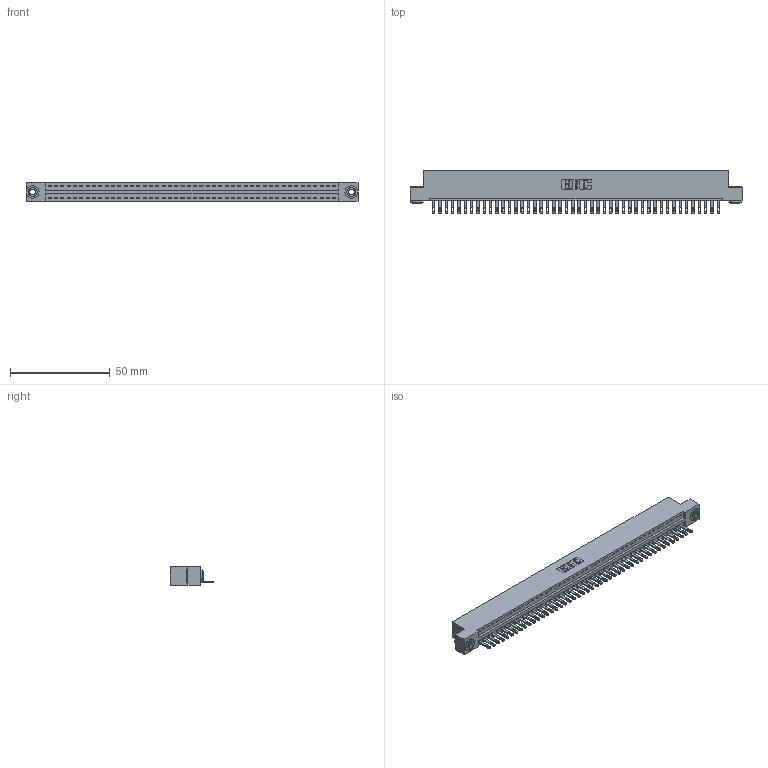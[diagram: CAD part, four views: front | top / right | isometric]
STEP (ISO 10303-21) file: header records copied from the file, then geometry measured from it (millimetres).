
FILE_DESCRIPTION (( 'STEP AP203' ), '1' );
FILE_NAME ('346-046-500-103.STEP', '2018-08-25T04:23:24', ( '' ), ( '' ), 'SwSTEP 2.0', 'SolidWorks 2016', '' );
FILE_SCHEMA (( 'CONFIG_CONTROL_DESIGN' ));
Length unit declared in the file: inch
Products named in the file (4): 346 Part_Flush Mounting Lugs - 0.156 Dia-TH; 345-292-001_345-293-100; 345-250-002_345-250-002-102; 346-046-500-103
Assembly tree (49 placements, depth 2):
  346-046-500-103
    346 Part_Flush Mounting Lugs - 0.156 Dia-TH
    345-292-001_345-293-100  x46
    345-250-002_345-250-002-102  x2
Bounding box: 166.62 x 21.84 x 9.4 mm (x, y, z)
Volume: 16025 mm3; surface area: 20398.7 mm2
Topology: 49 solids, 49 shells, 2644 faces, 8133 edges, 5418 vertices
Faces by surface type: plane 1650, cylinder 986, cone 8
Entity records: 28590 total; most frequent: CARTESIAN_POINT 4877, ORIENTED_EDGE 4850, DIRECTION 4331, EDGE_CURVE 2425, VECTOR 2081, LINE 2081, VERTEX_POINT 1614, AXIS2_PLACEMENT_3D 1125
